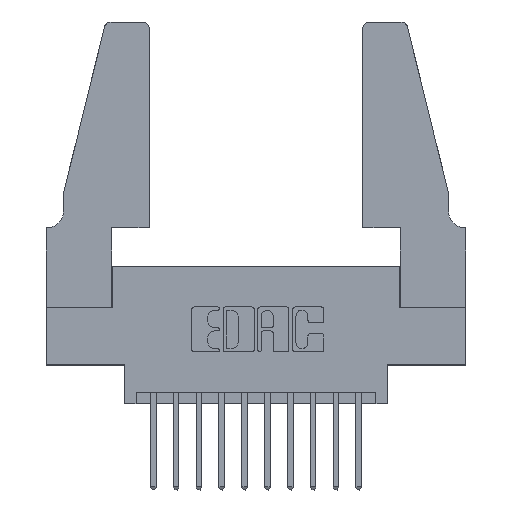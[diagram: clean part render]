
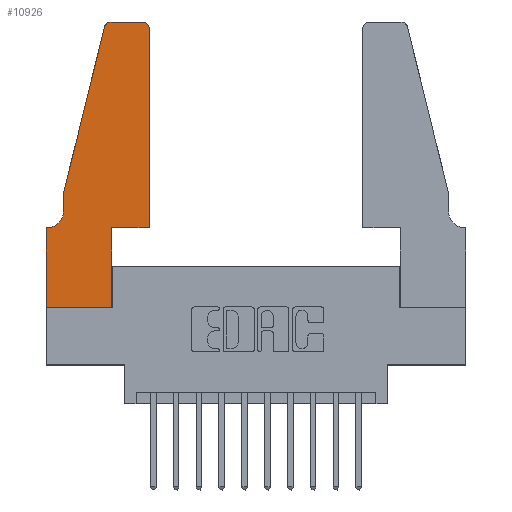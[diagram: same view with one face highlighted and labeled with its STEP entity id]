
A CAD part, top view. The second image highlights one B-rep face of the part: STEP entity #10926.
In plain terms, the highlighted planar face has unit normal (0, 0, 1).
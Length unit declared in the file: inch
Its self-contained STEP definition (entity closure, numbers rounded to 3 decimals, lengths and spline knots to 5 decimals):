
#230 = EDGE_CURVE ( 'NONE', #5821, #540, #9994, .T. ) ;
#301 = EDGE_CURVE ( 'NONE', #2111, #5821, #5973, .T. ) ;
#484 = ORIENTED_EDGE ( 'NONE', *, *, #8773, .T. ) ;
#540 = VERTEX_POINT ( 'NONE', #3722 ) ;
#544 = CARTESIAN_POINT ( 'NONE',  ( 0., 0., 0.37 ) ) ;
#574 = CIRCLE ( 'NONE', #8269, 0.03 ) ;
#624 = DIRECTION ( 'NONE',  ( -1., 0., 0. ) ) ;
#748 = EDGE_CURVE ( 'NONE', #3434, #7394, #574, .T. ) ;
#808 = CARTESIAN_POINT ( 'NONE',  ( 0., 0., 0.37 ) ) ;
#826 = ORIENTED_EDGE ( 'NONE', *, *, #13405, .T. ) ;
#842 = EDGE_CURVE ( 'NONE', #10986, #8080, #11153, .T. ) ;
#935 = CARTESIAN_POINT ( 'NONE',  ( 0.4505, 1.22, 0.37 ) ) ;
#1019 = CARTESIAN_POINT ( 'NONE',  ( 0.0755, 0.42, 0.37 ) ) ;
#1106 = DIRECTION ( 'NONE',  ( 0., 0., 1. ) ) ;
#1254 = CARTESIAN_POINT ( 'NONE',  ( 0.4505, 0.35, 0.37 ) ) ;
#1396 = EDGE_CURVE ( 'NONE', #2312, #3434, #13330, .T. ) ;
#1622 = VECTOR ( 'NONE', #2441, 39.37008 ) ;
#1726 = VERTEX_POINT ( 'NONE', #11067 ) ;
#1961 = LINE ( 'NONE', #12746, #13091 ) ;
#2064 = ORIENTED_EDGE ( 'NONE', *, *, #3048, .T. ) ;
#2111 = VERTEX_POINT ( 'NONE', #808 ) ;
#2312 = VERTEX_POINT ( 'NONE', #9171 ) ;
#2441 = DIRECTION ( 'NONE',  ( 1., 0., 0. ) ) ;
#2993 = VECTOR ( 'NONE', #5000, 39.37008 ) ;
#3048 = EDGE_CURVE ( 'NONE', #540, #2312, #8004, .T. ) ;
#3434 = VERTEX_POINT ( 'NONE', #935 ) ;
#3508 = DIRECTION ( 'NONE',  ( 0., 0., 1. ) ) ;
#3529 = CARTESIAN_POINT ( 'NONE',  ( 0.4205, 1.22, 0.37 ) ) ;
#3647 = DIRECTION ( 'NONE',  ( 0., -1., 0. ) ) ;
#3704 = CARTESIAN_POINT ( 'NONE',  ( 0.25487, 1.22718, 0.37 ) ) ;
#3722 = CARTESIAN_POINT ( 'NONE',  ( 0.2865, 0.35, 0.37 ) ) ;
#3901 = VERTEX_POINT ( 'NONE', #8595 ) ;
#4165 = LINE ( 'NONE', #6342, #9750 ) ;
#4450 = CARTESIAN_POINT ( 'NONE',  ( 0.4505, 0.35, 0.37 ) ) ;
#4728 = VERTEX_POINT ( 'NONE', #8924 ) ;
#5000 = DIRECTION ( 'NONE',  ( 1., 0., 0. ) ) ;
#5054 = DIRECTION ( 'NONE',  ( -1., 0., 0. ) ) ;
#5693 = CIRCLE ( 'NONE', #6735, 0.07 ) ;
#5749 = DIRECTION ( 'NONE',  ( 0., 1., 0. ) ) ;
#5821 = VERTEX_POINT ( 'NONE', #10958 ) ;
#5967 = FACE_OUTER_BOUND ( 'NONE', #11029, .T. ) ;
#5969 = CARTESIAN_POINT ( 'NONE',  ( 0.0755, 0.5, 0.37 ) ) ;
#5973 = LINE ( 'NONE', #6641, #2993 ) ;
#6000 = CARTESIAN_POINT ( 'NONE',  ( 0.2865, 0.35, 0.37 ) ) ;
#6024 = AXIS2_PLACEMENT_3D ( 'NONE', #13171, #6599, #14235 ) ;
#6342 = CARTESIAN_POINT ( 'NONE',  ( 0.0755, 0.35, 0.37 ) ) ;
#6570 = VERTEX_POINT ( 'NONE', #3704 ) ;
#6593 = ORIENTED_EDGE ( 'NONE', *, *, #1396, .T. ) ;
#6599 = DIRECTION ( 'NONE',  ( 0., 0., 1. ) ) ;
#6641 = CARTESIAN_POINT ( 'NONE',  ( 0., 0., 0.37 ) ) ;
#6735 = AXIS2_PLACEMENT_3D ( 'NONE', #13304, #6743, #14367 ) ;
#6743 = DIRECTION ( 'NONE',  ( 0., 0., -1. ) ) ;
#6801 = ORIENTED_EDGE ( 'NONE', *, *, #301, .T. ) ;
#6952 = AXIS2_PLACEMENT_3D ( 'NONE', #7931, #1106, #9066 ) ;
#7393 = DIRECTION ( 'NONE',  ( 0., -1., 0. ) ) ;
#7394 = VERTEX_POINT ( 'NONE', #8258 ) ;
#7737 = VECTOR ( 'NONE', #7393, 39.37008 ) ;
#7839 = PLANE ( 'NONE',  #6952 ) ;
#7931 = CARTESIAN_POINT ( 'NONE',  ( 0., 0.35, 0.37 ) ) ;
#8004 = LINE ( 'NONE', #1254, #1622 ) ;
#8080 = VERTEX_POINT ( 'NONE', #1019 ) ;
#8252 = VECTOR ( 'NONE', #3647, 39.37008 ) ;
#8258 = CARTESIAN_POINT ( 'NONE',  ( 0.4205, 1.25, 0.37 ) ) ;
#8269 = AXIS2_PLACEMENT_3D ( 'NONE', #3529, #3508, #9182 ) ;
#8423 = EDGE_CURVE ( 'NONE', #7394, #3901, #1961, .T. ) ;
#8595 = CARTESIAN_POINT ( 'NONE',  ( 0.284, 1.25, 0.37 ) ) ;
#8773 = EDGE_CURVE ( 'NONE', #8080, #4728, #5693, .T. ) ;
#8782 = ORIENTED_EDGE ( 'NONE', *, *, #12742, .T. ) ;
#8924 = CARTESIAN_POINT ( 'NONE',  ( 0.0055, 0.35, 0.37 ) ) ;
#9066 = DIRECTION ( 'NONE',  ( 1., 0., 0. ) ) ;
#9101 = DIRECTION ( 'NONE',  ( -0.239, -0.971, 0. ) ) ;
#9171 = CARTESIAN_POINT ( 'NONE',  ( 0.4505, 0.35, 0.37 ) ) ;
#9182 = DIRECTION ( 'NONE',  ( 1., 0., 0. ) ) ;
#9239 = ORIENTED_EDGE ( 'NONE', *, *, #842, .T. ) ;
#9660 = VECTOR ( 'NONE', #5749, 39.37008 ) ;
#9735 = DIRECTION ( 'NONE',  ( 0., 1., 0. ) ) ;
#9750 = VECTOR ( 'NONE', #624, 39.37008 ) ;
#9994 = LINE ( 'NONE', #6000, #9660 ) ;
#10233 = CIRCLE ( 'NONE', #6024, 0.03 ) ;
#10359 = EDGE_CURVE ( 'NONE', #1726, #2111, #10996, .T. ) ;
#10435 = ORIENTED_EDGE ( 'NONE', *, *, #10359, .T. ) ;
#10447 = VECTOR ( 'NONE', #9735, 39.37008 ) ;
#10913 = LINE ( 'NONE', #14451, #13107 ) ;
#10926 = ADVANCED_FACE ( 'NONE', ( #5967 ), #7839, .T. ) ;
#10958 = CARTESIAN_POINT ( 'NONE',  ( 0.2865, 0., 0.37 ) ) ;
#10986 = VERTEX_POINT ( 'NONE', #13398 ) ;
#10996 = LINE ( 'NONE', #544, #7737 ) ;
#11029 = EDGE_LOOP ( 'NONE', ( #14077, #8782, #826, #9239, #484, #11925, #10435, #6801, #11634, #2064, #6593, #14354 ) ) ;
#11067 = CARTESIAN_POINT ( 'NONE',  ( 0., 0.35, 0.37 ) ) ;
#11153 = LINE ( 'NONE', #5969, #8252 ) ;
#11634 = ORIENTED_EDGE ( 'NONE', *, *, #230, .T. ) ;
#11925 = ORIENTED_EDGE ( 'NONE', *, *, #13224, .T. ) ;
#12742 = EDGE_CURVE ( 'NONE', #3901, #6570, #10233, .T. ) ;
#12746 = CARTESIAN_POINT ( 'NONE',  ( 0.2605, 1.25, 0.37 ) ) ;
#13091 = VECTOR ( 'NONE', #5054, 39.37008 ) ;
#13107 = VECTOR ( 'NONE', #9101, 39.37008 ) ;
#13171 = CARTESIAN_POINT ( 'NONE',  ( 0.284, 1.22, 0.37 ) ) ;
#13224 = EDGE_CURVE ( 'NONE', #4728, #1726, #4165, .T. ) ;
#13304 = CARTESIAN_POINT ( 'NONE',  ( 0.0055, 0.42, 0.37 ) ) ;
#13330 = LINE ( 'NONE', #4450, #10447 ) ;
#13398 = CARTESIAN_POINT ( 'NONE',  ( 0.0755, 0.5, 0.37 ) ) ;
#13405 = EDGE_CURVE ( 'NONE', #6570, #10986, #10913, .T. ) ;
#14077 = ORIENTED_EDGE ( 'NONE', *, *, #8423, .T. ) ;
#14235 = DIRECTION ( 'NONE',  ( 1., 0., 0. ) ) ;
#14354 = ORIENTED_EDGE ( 'NONE', *, *, #748, .T. ) ;
#14367 = DIRECTION ( 'NONE',  ( -1., 0., 0. ) ) ;
#14451 = CARTESIAN_POINT ( 'NONE',  ( 0.0755, 0.5, 0.37 ) ) ;
